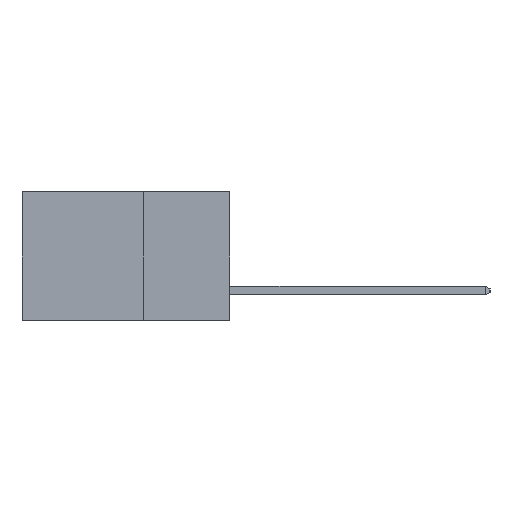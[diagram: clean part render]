
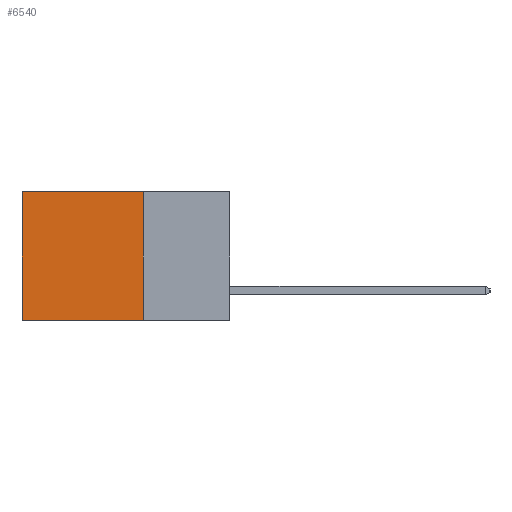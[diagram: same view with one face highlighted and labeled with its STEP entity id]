
A CAD part, left-side view. The second image highlights one B-rep face of the part: STEP entity #6540.
In plain terms, the highlighted planar face has unit normal (-1, 0, 0).
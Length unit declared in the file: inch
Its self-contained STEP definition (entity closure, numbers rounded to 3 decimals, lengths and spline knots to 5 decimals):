
#174 = LINE ( 'NONE', #9163, #4467 ) ;
#361 = AXIS2_PLACEMENT_3D ( 'NONE', #9323, #9318, #9251 ) ;
#1300 = LINE ( 'NONE', #14719, #5676 ) ;
#2050 = CARTESIAN_POINT ( 'NONE',  ( 0.2615, 0.6, 0. ) ) ;
#2148 = ORIENTED_EDGE ( 'NONE', *, *, #10822, .T. ) ;
#3064 = DIRECTION ( 'NONE',  ( 0., 0., -1. ) ) ;
#3188 = CARTESIAN_POINT ( 'NONE',  ( 0.2615, 0.25, -0.37 ) ) ;
#3907 = EDGE_CURVE ( 'NONE', #11576, #6062, #1300, .T. ) ;
#4467 = VECTOR ( 'NONE', #9156, 39.37008 ) ;
#5519 = CARTESIAN_POINT ( 'NONE',  ( 0.2615, 0.25, -0.37 ) ) ;
#5676 = VECTOR ( 'NONE', #14910, 39.37008 ) ;
#6062 = VERTEX_POINT ( 'NONE', #6340 ) ;
#6340 = CARTESIAN_POINT ( 'NONE',  ( 0.2615, 0.6, -0.37 ) ) ;
#6540 = ADVANCED_FACE ( 'NONE', ( #14658 ), #9908, .F. ) ;
#6747 = ORIENTED_EDGE ( 'NONE', *, *, #3907, .F. ) ;
#7215 = CARTESIAN_POINT ( 'NONE',  ( 0.2615, 0.25, 0. ) ) ;
#8388 = EDGE_CURVE ( 'NONE', #17385, #6062, #174, .T. ) ;
#9059 = EDGE_LOOP ( 'NONE', ( #11014, #6747, #17606, #2148 ) ) ;
#9156 = DIRECTION ( 'NONE',  ( 0., 0., -1. ) ) ;
#9163 = CARTESIAN_POINT ( 'NONE',  ( 0.2615, 0.6, -0.37 ) ) ;
#9251 = DIRECTION ( 'NONE',  ( 0., 0., -1. ) ) ;
#9318 = DIRECTION ( 'NONE',  ( 1., 0., 0. ) ) ;
#9323 = CARTESIAN_POINT ( 'NONE',  ( 0.2615, 0.25, -0.37 ) ) ;
#9541 = LINE ( 'NONE', #3188, #13291 ) ;
#9908 = PLANE ( 'NONE',  #361 ) ;
#10822 = EDGE_CURVE ( 'NONE', #11374, #17385, #15492, .T. ) ;
#11014 = ORIENTED_EDGE ( 'NONE', *, *, #8388, .T. ) ;
#11374 = VERTEX_POINT ( 'NONE', #7215 ) ;
#11576 = VERTEX_POINT ( 'NONE', #5519 ) ;
#12882 = CARTESIAN_POINT ( 'NONE',  ( 0.2615, 0.25, 0. ) ) ;
#12902 = DIRECTION ( 'NONE',  ( 0., 1., 0. ) ) ;
#13291 = VECTOR ( 'NONE', #3064, 39.37008 ) ;
#14658 = FACE_OUTER_BOUND ( 'NONE', #9059, .T. ) ;
#14719 = CARTESIAN_POINT ( 'NONE',  ( 0.2615, 0.25, -0.37 ) ) ;
#14910 = DIRECTION ( 'NONE',  ( 0., 1., 0. ) ) ;
#15023 = VECTOR ( 'NONE', #12902, 39.37008 ) ;
#15492 = LINE ( 'NONE', #12882, #15023 ) ;
#17335 = EDGE_CURVE ( 'NONE', #11374, #11576, #9541, .T. ) ;
#17385 = VERTEX_POINT ( 'NONE', #2050 ) ;
#17606 = ORIENTED_EDGE ( 'NONE', *, *, #17335, .F. ) ;
